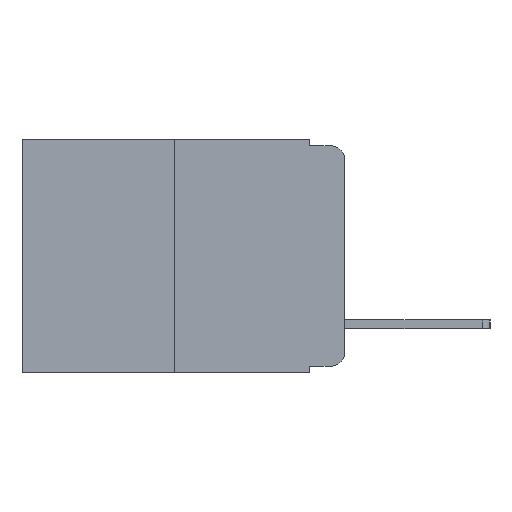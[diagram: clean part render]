
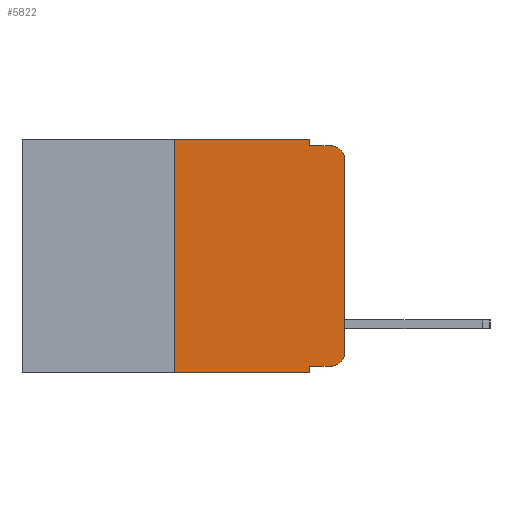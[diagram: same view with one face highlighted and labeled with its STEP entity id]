
A CAD part, left-side view. The second image highlights one B-rep face of the part: STEP entity #5822.
In plain terms, the highlighted planar face has unit normal (-1, 0, 0).
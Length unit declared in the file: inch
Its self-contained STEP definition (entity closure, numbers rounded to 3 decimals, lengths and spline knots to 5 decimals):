
#859 = VERTEX_POINT ( 'NONE', #20795 ) ;
#1007 = VECTOR ( 'NONE', #12577, 39.37008 ) ;
#1552 = VECTOR ( 'NONE', #9930, 39.37008 ) ;
#1619 = LINE ( 'NONE', #10750, #1007 ) ;
#2013 = EDGE_LOOP ( 'NONE', ( #18613, #16045, #5849, #13335, #11125, #10720, #9026, #12754, #21611, #18068 ) ) ;
#2362 = DIRECTION ( 'NONE',  ( 0., -1., 0. ) ) ;
#2730 = VECTOR ( 'NONE', #16391, 39.37008 ) ;
#4105 = DIRECTION ( 'NONE',  ( 0., -1., 0. ) ) ;
#5329 = CARTESIAN_POINT ( 'NONE',  ( 0., 0.051, -0.01 ) ) ;
#5580 = CARTESIAN_POINT ( 'NONE',  ( 0., 0.25, -0.343 ) ) ;
#5700 = DIRECTION ( 'NONE',  ( 0., 0., -1. ) ) ;
#5822 = ADVANCED_FACE ( 'NONE', ( #24003 ), #9415, .F. ) ;
#5849 = ORIENTED_EDGE ( 'NONE', *, *, #18415, .F. ) ;
#6291 = EDGE_CURVE ( 'NONE', #11586, #17561, #23979, .T. ) ;
#6499 = CARTESIAN_POINT ( 'NONE',  ( 0., 0.02, -0.01 ) ) ;
#7748 = DIRECTION ( 'NONE',  ( 0., 0., -1. ) ) ;
#7910 = VERTEX_POINT ( 'NONE', #5580 ) ;
#8065 = CARTESIAN_POINT ( 'NONE',  ( 0., 0., 0. ) ) ;
#8228 = LINE ( 'NONE', #11074, #22148 ) ;
#8821 = CARTESIAN_POINT ( 'NONE',  ( 0., 0.02, -0.03 ) ) ;
#8995 = DIRECTION ( 'NONE',  ( 0., 0., -1. ) ) ;
#9026 = ORIENTED_EDGE ( 'NONE', *, *, #13261, .T. ) ;
#9415 = PLANE ( 'NONE',  #17718 ) ;
#9622 = CARTESIAN_POINT ( 'NONE',  ( 0., 0.051, 0. ) ) ;
#9930 = DIRECTION ( 'NONE',  ( 0., 0., 1. ) ) ;
#10029 = CARTESIAN_POINT ( 'NONE',  ( 0., 0.02, -0.313 ) ) ;
#10145 = CARTESIAN_POINT ( 'NONE',  ( 0., 0., -0.03 ) ) ;
#10660 = DIRECTION ( 'NONE',  ( 0., 0., -1. ) ) ;
#10720 = ORIENTED_EDGE ( 'NONE', *, *, #15106, .F. ) ;
#10750 = CARTESIAN_POINT ( 'NONE',  ( 0., 0.051, -0.01 ) ) ;
#11074 = CARTESIAN_POINT ( 'NONE',  ( 0., 0.473, 0. ) ) ;
#11125 = ORIENTED_EDGE ( 'NONE', *, *, #18549, .F. ) ;
#11586 = VERTEX_POINT ( 'NONE', #19715 ) ;
#11879 = DIRECTION ( 'NONE',  ( 0., 0., -1. ) ) ;
#12467 = CIRCLE ( 'NONE', #17810, 0.02 ) ;
#12577 = DIRECTION ( 'NONE',  ( 0., -1., 0. ) ) ;
#12716 = LINE ( 'NONE', #23622, #2730 ) ;
#12754 = ORIENTED_EDGE ( 'NONE', *, *, #6291, .F. ) ;
#13238 = EDGE_CURVE ( 'NONE', #20112, #18890, #16482, .T. ) ;
#13261 = EDGE_CURVE ( 'NONE', #7910, #17561, #15932, .T. ) ;
#13335 = ORIENTED_EDGE ( 'NONE', *, *, #22754, .F. ) ;
#13585 = VERTEX_POINT ( 'NONE', #5329 ) ;
#14327 = LINE ( 'NONE', #15226, #23861 ) ;
#14439 = VECTOR ( 'NONE', #8995, 39.37008 ) ;
#14529 = EDGE_CURVE ( 'NONE', #18868, #20112, #12467, .T. ) ;
#14849 = VERTEX_POINT ( 'NONE', #6499 ) ;
#15106 = EDGE_CURVE ( 'NONE', #7910, #859, #12716, .T. ) ;
#15226 = CARTESIAN_POINT ( 'NONE',  ( 0., 0.051, -0.333 ) ) ;
#15471 = CARTESIAN_POINT ( 'NONE',  ( 0., 0.473, -0.343 ) ) ;
#15932 = LINE ( 'NONE', #15471, #21825 ) ;
#16045 = ORIENTED_EDGE ( 'NONE', *, *, #23672, .T. ) ;
#16284 = AXIS2_PLACEMENT_3D ( 'NONE', #8821, #21494, #10660 ) ;
#16391 = DIRECTION ( 'NONE',  ( 0., 0., 1. ) ) ;
#16482 = LINE ( 'NONE', #8065, #1552 ) ;
#16727 = DIRECTION ( 'NONE',  ( 1., 0., 0. ) ) ;
#17561 = VERTEX_POINT ( 'NONE', #23971 ) ;
#17679 = CIRCLE ( 'NONE', #16284, 0.02 ) ;
#17718 = AXIS2_PLACEMENT_3D ( 'NONE', #23883, #16727, #5700 ) ;
#17810 = AXIS2_PLACEMENT_3D ( 'NONE', #10029, #22683, #11879 ) ;
#18068 = ORIENTED_EDGE ( 'NONE', *, *, #14529, .T. ) ;
#18415 = EDGE_CURVE ( 'NONE', #13585, #14849, #1619, .T. ) ;
#18549 = EDGE_CURVE ( 'NONE', #859, #19378, #8228, .T. ) ;
#18613 = ORIENTED_EDGE ( 'NONE', *, *, #13238, .T. ) ;
#18849 = VECTOR ( 'NONE', #7748, 39.37008 ) ;
#18868 = VERTEX_POINT ( 'NONE', #22805 ) ;
#18890 = VERTEX_POINT ( 'NONE', #10145 ) ;
#19311 = CARTESIAN_POINT ( 'NONE',  ( 0., 0., -0.313 ) ) ;
#19378 = VERTEX_POINT ( 'NONE', #22313 ) ;
#19414 = LINE ( 'NONE', #9622, #18849 ) ;
#19715 = CARTESIAN_POINT ( 'NONE',  ( 0., 0.051, -0.333 ) ) ;
#20090 = DIRECTION ( 'NONE',  ( 0., -1., 0. ) ) ;
#20112 = VERTEX_POINT ( 'NONE', #19311 ) ;
#20795 = CARTESIAN_POINT ( 'NONE',  ( 0., 0.25, 0. ) ) ;
#21494 = DIRECTION ( 'NONE',  ( -1., 0., 0. ) ) ;
#21611 = ORIENTED_EDGE ( 'NONE', *, *, #23398, .T. ) ;
#21668 = CARTESIAN_POINT ( 'NONE',  ( 0., 0.051, 0. ) ) ;
#21825 = VECTOR ( 'NONE', #2362, 39.37008 ) ;
#22148 = VECTOR ( 'NONE', #20090, 39.37008 ) ;
#22313 = CARTESIAN_POINT ( 'NONE',  ( 0., 0.051, 0. ) ) ;
#22683 = DIRECTION ( 'NONE',  ( -1., 0., 0. ) ) ;
#22754 = EDGE_CURVE ( 'NONE', #19378, #13585, #19414, .T. ) ;
#22805 = CARTESIAN_POINT ( 'NONE',  ( 0., 0.02, -0.333 ) ) ;
#23398 = EDGE_CURVE ( 'NONE', #11586, #18868, #14327, .T. ) ;
#23622 = CARTESIAN_POINT ( 'NONE',  ( 0., 0.25, 0. ) ) ;
#23672 = EDGE_CURVE ( 'NONE', #18890, #14849, #17679, .T. ) ;
#23861 = VECTOR ( 'NONE', #4105, 39.37008 ) ;
#23883 = CARTESIAN_POINT ( 'NONE',  ( 0., 0.473, 0. ) ) ;
#23971 = CARTESIAN_POINT ( 'NONE',  ( 0., 0.051, -0.343 ) ) ;
#23979 = LINE ( 'NONE', #21668, #14439 ) ;
#24003 = FACE_OUTER_BOUND ( 'NONE', #2013, .T. ) ;
